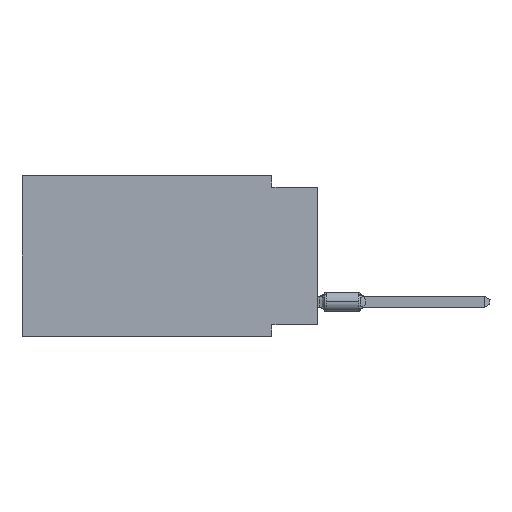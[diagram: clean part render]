
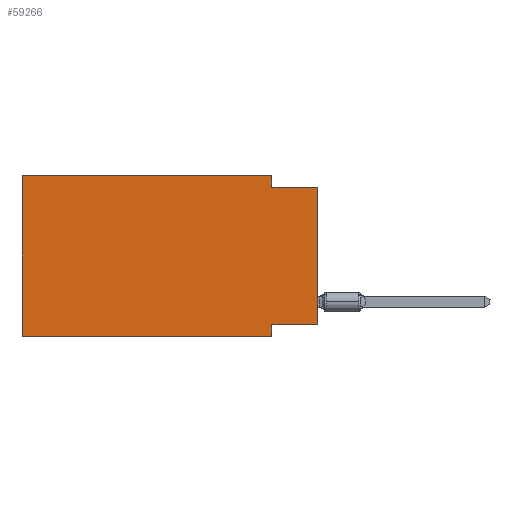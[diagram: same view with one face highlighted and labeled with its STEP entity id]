
A CAD part, left-side view. The second image highlights one B-rep face of the part: STEP entity #59266.
In plain terms, the highlighted planar face has unit normal (-1, 0, 0).
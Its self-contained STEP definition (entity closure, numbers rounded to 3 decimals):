
#178 = DIRECTION ( 'NONE',  ( 0., 1., 0. ) ) ;
#757 = VECTOR ( 'NONE', #31209, 1000. ) ;
#2322 = CARTESIAN_POINT ( 'NONE',  ( 0., 0., -8.255 ) ) ;
#2815 = CARTESIAN_POINT ( 'NONE',  ( 0., 16.383, 0. ) ) ;
#2964 = VERTEX_POINT ( 'NONE', #18551 ) ;
#3376 = ORIENTED_EDGE ( 'NONE', *, *, #70923, .F. ) ;
#3448 = EDGE_CURVE ( 'NONE', #54444, #76581, #75629, .T. ) ;
#3799 = VECTOR ( 'NONE', #75803, 1000. ) ;
#4826 = CARTESIAN_POINT ( 'NONE',  ( 0., 16.383, 0. ) ) ;
#5041 = LINE ( 'NONE', #33427, #22990 ) ;
#5844 = CARTESIAN_POINT ( 'NONE',  ( 0., 16.383, 0. ) ) ;
#5926 = VECTOR ( 'NONE', #68249, 1000. ) ;
#10568 = EDGE_CURVE ( 'NONE', #76581, #87828, #59177, .T. ) ;
#11345 = DIRECTION ( 'NONE',  ( 0., 0., -1. ) ) ;
#11822 = DIRECTION ( 'NONE',  ( 0., 0., 1. ) ) ;
#12117 = CARTESIAN_POINT ( 'NONE',  ( 0., 2.54, 0. ) ) ;
#15734 = ORIENTED_EDGE ( 'NONE', *, *, #3448, .F. ) ;
#17176 = DIRECTION ( 'NONE',  ( 0., -1., 0. ) ) ;
#18551 = CARTESIAN_POINT ( 'NONE',  ( 0., 2.54, -0.635 ) ) ;
#18855 = VECTOR ( 'NONE', #74555, 1000. ) ;
#19339 = CARTESIAN_POINT ( 'NONE',  ( 0., 0., 0. ) ) ;
#21128 = CARTESIAN_POINT ( 'NONE',  ( 0., 0., -8.255 ) ) ;
#21797 = VECTOR ( 'NONE', #178, 1000. ) ;
#22990 = VECTOR ( 'NONE', #17176, 1000. ) ;
#25133 = EDGE_LOOP ( 'NONE', ( #43544, #29029, #88482, #68558, #15734, #76698, #3376, #39746 ) ) ;
#25315 = CARTESIAN_POINT ( 'NONE',  ( 0., 2.54, -8.89 ) ) ;
#26993 = LINE ( 'NONE', #12117, #18855 ) ;
#28041 = PLANE ( 'NONE',  #51718 ) ;
#29029 = ORIENTED_EDGE ( 'NONE', *, *, #84164, .F. ) ;
#29335 = CARTESIAN_POINT ( 'NONE',  ( 0., 2.54, 0. ) ) ;
#30918 = LINE ( 'NONE', #25315, #61779 ) ;
#31209 = DIRECTION ( 'NONE',  ( 0., -1., 0. ) ) ;
#33427 = CARTESIAN_POINT ( 'NONE',  ( 0., 16.383, -8.89 ) ) ;
#33484 = EDGE_CURVE ( 'NONE', #74384, #84449, #35996, .T. ) ;
#35552 = VECTOR ( 'NONE', #11822, 1000. ) ;
#35996 = LINE ( 'NONE', #21128, #21797 ) ;
#36071 = EDGE_CURVE ( 'NONE', #54444, #50639, #5041, .T. ) ;
#39746 = ORIENTED_EDGE ( 'NONE', *, *, #33484, .F. ) ;
#43544 = ORIENTED_EDGE ( 'NONE', *, *, #50909, .T. ) ;
#44013 = VERTEX_POINT ( 'NONE', #62552 ) ;
#46828 = LINE ( 'NONE', #19339, #5926 ) ;
#48081 = CARTESIAN_POINT ( 'NONE',  ( 0., 16.383, 0. ) ) ;
#50639 = VERTEX_POINT ( 'NONE', #71145 ) ;
#50909 = EDGE_CURVE ( 'NONE', #74384, #44013, #46828, .T. ) ;
#51718 = AXIS2_PLACEMENT_3D ( 'NONE', #48081, #63460, #76507 ) ;
#54444 = VERTEX_POINT ( 'NONE', #58971 ) ;
#58971 = CARTESIAN_POINT ( 'NONE',  ( 0., 16.383, -8.89 ) ) ;
#59177 = LINE ( 'NONE', #2815, #757 ) ;
#59266 = ADVANCED_FACE ( 'NONE', ( #83467 ), #28041, .F. ) ;
#61779 = VECTOR ( 'NONE', #11345, 1000. ) ;
#62139 = EDGE_CURVE ( 'NONE', #87828, #2964, #26993, .T. ) ;
#62277 = LINE ( 'NONE', #67429, #3799 ) ;
#62552 = CARTESIAN_POINT ( 'NONE',  ( 0., 0., -0.635 ) ) ;
#63460 = DIRECTION ( 'NONE',  ( 1., 0., 0. ) ) ;
#65491 = CARTESIAN_POINT ( 'NONE',  ( 0., 2.54, -8.255 ) ) ;
#67429 = CARTESIAN_POINT ( 'NONE',  ( 0., 0., -0.635 ) ) ;
#68249 = DIRECTION ( 'NONE',  ( 0., 0., 1. ) ) ;
#68558 = ORIENTED_EDGE ( 'NONE', *, *, #10568, .F. ) ;
#70923 = EDGE_CURVE ( 'NONE', #84449, #50639, #30918, .T. ) ;
#71145 = CARTESIAN_POINT ( 'NONE',  ( 0., 2.54, -8.89 ) ) ;
#74384 = VERTEX_POINT ( 'NONE', #2322 ) ;
#74555 = DIRECTION ( 'NONE',  ( 0., 0., -1. ) ) ;
#75629 = LINE ( 'NONE', #4826, #35552 ) ;
#75803 = DIRECTION ( 'NONE',  ( 0., -1., 0. ) ) ;
#76507 = DIRECTION ( 'NONE',  ( 0., 0., -1. ) ) ;
#76581 = VERTEX_POINT ( 'NONE', #5844 ) ;
#76698 = ORIENTED_EDGE ( 'NONE', *, *, #36071, .T. ) ;
#83467 = FACE_OUTER_BOUND ( 'NONE', #25133, .T. ) ;
#84164 = EDGE_CURVE ( 'NONE', #2964, #44013, #62277, .T. ) ;
#84449 = VERTEX_POINT ( 'NONE', #65491 ) ;
#87828 = VERTEX_POINT ( 'NONE', #29335 ) ;
#88482 = ORIENTED_EDGE ( 'NONE', *, *, #62139, .F. ) ;
